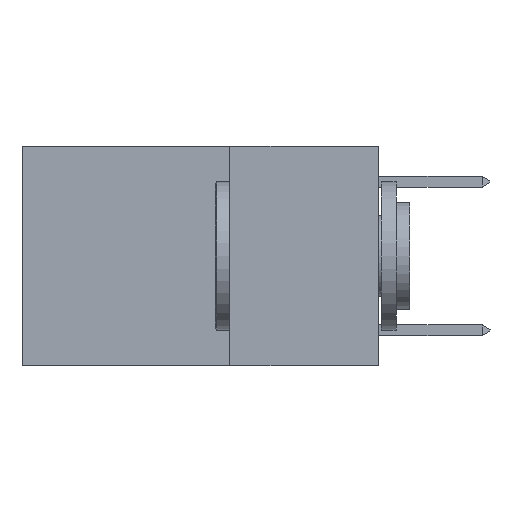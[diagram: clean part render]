
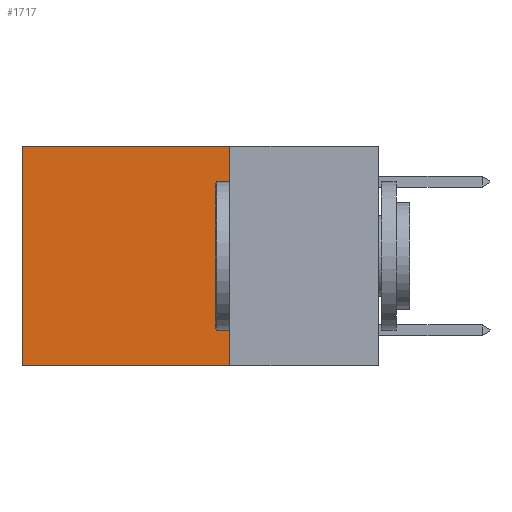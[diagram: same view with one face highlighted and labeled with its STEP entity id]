
A CAD part, left-side view. The second image highlights one B-rep face of the part: STEP entity #1717.
In plain terms, the highlighted planar face has unit normal (-1, 0, 0).
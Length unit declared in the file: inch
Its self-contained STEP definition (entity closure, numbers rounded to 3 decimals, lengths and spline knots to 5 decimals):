
#597 = EDGE_LOOP ( 'NONE', ( #18527, #17324, #16657, #13477 ) ) ;
#1717 = ADVANCED_FACE ( 'NONE', ( #5330 ), #18455, .F. ) ;
#1892 = EDGE_CURVE ( 'NONE', #16123, #10868, #21160, .T. ) ;
#2352 = VERTEX_POINT ( 'NONE', #22697 ) ;
#3187 = AXIS2_PLACEMENT_3D ( 'NONE', #16912, #15304, #15218 ) ;
#4057 = LINE ( 'NONE', #13273, #5333 ) ;
#4913 = CARTESIAN_POINT ( 'NONE',  ( 0.2625, 0.25, -0.37 ) ) ;
#5330 = FACE_OUTER_BOUND ( 'NONE', #597, .T. ) ;
#5333 = VECTOR ( 'NONE', #12791, 39.37008 ) ;
#7261 = LINE ( 'NONE', #16420, #8467 ) ;
#8467 = VECTOR ( 'NONE', #17111, 39.37008 ) ;
#9172 = VECTOR ( 'NONE', #18118, 39.37008 ) ;
#9308 = LINE ( 'NONE', #18148, #9172 ) ;
#10868 = VERTEX_POINT ( 'NONE', #19067 ) ;
#11401 = CARTESIAN_POINT ( 'NONE',  ( 0.2625, 0.25, -0.37 ) ) ;
#12791 = DIRECTION ( 'NONE',  ( 0., 0., -1. ) ) ;
#13273 = CARTESIAN_POINT ( 'NONE',  ( 0.2625, 0.25, 0. ) ) ;
#13477 = ORIENTED_EDGE ( 'NONE', *, *, #19336, .T. ) ;
#15046 = VECTOR ( 'NONE', #24399, 39.37008 ) ;
#15218 = DIRECTION ( 'NONE',  ( 0., 0., -1. ) ) ;
#15304 = DIRECTION ( 'NONE',  ( 1., 0., 0. ) ) ;
#15998 = VERTEX_POINT ( 'NONE', #22825 ) ;
#16123 = VERTEX_POINT ( 'NONE', #4913 ) ;
#16420 = CARTESIAN_POINT ( 'NONE',  ( 0.2625, 0.6, 0. ) ) ;
#16657 = ORIENTED_EDGE ( 'NONE', *, *, #19498, .F. ) ;
#16912 = CARTESIAN_POINT ( 'NONE',  ( 0.2625, 0.25, 0. ) ) ;
#17111 = DIRECTION ( 'NONE',  ( 0., 0., -1. ) ) ;
#17324 = ORIENTED_EDGE ( 'NONE', *, *, #1892, .F. ) ;
#18118 = DIRECTION ( 'NONE',  ( 0., 1., 0. ) ) ;
#18148 = CARTESIAN_POINT ( 'NONE',  ( 0.2625, 0.25, 0. ) ) ;
#18455 = PLANE ( 'NONE',  #3187 ) ;
#18527 = ORIENTED_EDGE ( 'NONE', *, *, #18611, .T. ) ;
#18611 = EDGE_CURVE ( 'NONE', #15998, #10868, #7261, .T. ) ;
#19067 = CARTESIAN_POINT ( 'NONE',  ( 0.2625, 0.6, -0.37 ) ) ;
#19336 = EDGE_CURVE ( 'NONE', #2352, #15998, #9308, .T. ) ;
#19498 = EDGE_CURVE ( 'NONE', #2352, #16123, #4057, .T. ) ;
#21160 = LINE ( 'NONE', #11401, #15046 ) ;
#22697 = CARTESIAN_POINT ( 'NONE',  ( 0.2625, 0.25, 0. ) ) ;
#22825 = CARTESIAN_POINT ( 'NONE',  ( 0.2625, 0.6, 0. ) ) ;
#24399 = DIRECTION ( 'NONE',  ( 0., 1., 0. ) ) ;
